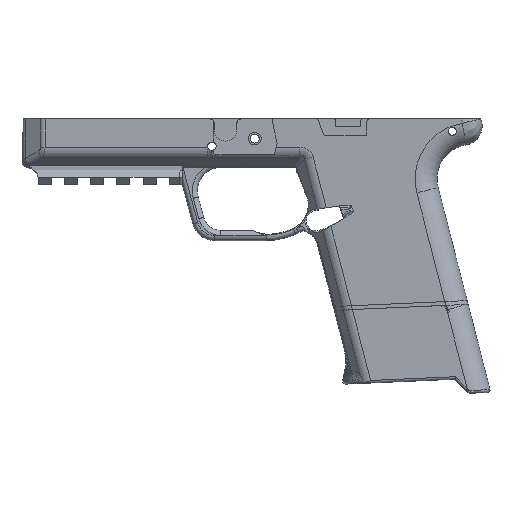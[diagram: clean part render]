
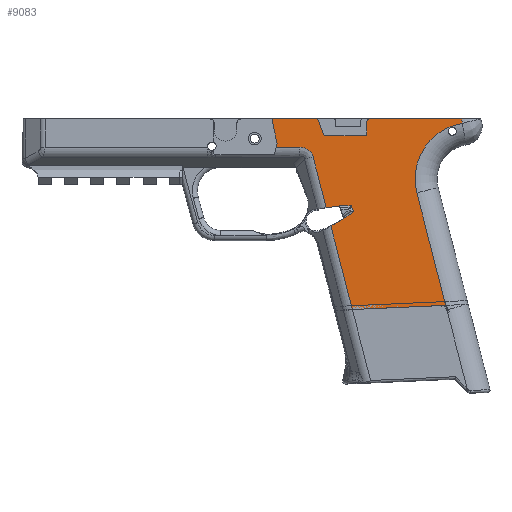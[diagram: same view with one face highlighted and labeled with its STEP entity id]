
A CAD part, left-side view. The second image highlights one B-rep face of the part: STEP entity #9083.
In plain terms, the highlighted face is planar.
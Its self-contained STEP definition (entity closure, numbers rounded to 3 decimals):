
#261=CIRCLE('',#9748,22.475);
#262=CIRCLE('',#9749,7.5);
#263=CIRCLE('',#9750,1.);
#264=CIRCLE('',#9751,1.);
#265=CIRCLE('',#9752,1.);
#266=CIRCLE('',#9753,1.);
#748=FACE_OUTER_BOUND('',#1268,.T.);
#1268=EDGE_LOOP('',(#6722,#6723,#6724,#6725,#6726,#6727,#6728,#6729,#6730,
#6731,#6732,#6733,#6734,#6735,#6736,#6737,#6738,#6739,#6740,#6741,#6742,
#6743,#6744,#6745,#6746,#6747));
#1880=LINE('',#14893,#2688);
#1882=LINE('',#14905,#2690);
#1884=LINE('',#14909,#2692);
#1895=LINE('',#14938,#2703);
#1896=LINE('',#14940,#2704);
#1897=LINE('',#14941,#2705);
#1898=LINE('',#14943,#2706);
#1899=LINE('',#14945,#2707);
#1900=LINE('',#14947,#2708);
#1901=LINE('',#14949,#2709);
#1902=LINE('',#14955,#2710);
#1903=LINE('',#14959,#2711);
#1904=LINE('',#14963,#2712);
#1905=LINE('',#14967,#2713);
#1906=LINE('',#14971,#2714);
#1907=LINE('',#14973,#2715);
#1908=LINE('',#14975,#2716);
#1909=LINE('',#14977,#2717);
#1910=LINE('',#14980,#2718);
#2688=VECTOR('',#11078,10.);
#2690=VECTOR('',#11088,10.);
#2692=VECTOR('',#11092,10.);
#2703=VECTOR('',#11113,10.);
#2704=VECTOR('',#11114,10.);
#2705=VECTOR('',#11115,10.);
#2706=VECTOR('',#11116,10.);
#2707=VECTOR('',#11117,10.);
#2708=VECTOR('',#11118,10.);
#2709=VECTOR('',#11119,10.);
#2710=VECTOR('',#11124,10.);
#2711=VECTOR('',#11127,10.);
#2712=VECTOR('',#11130,10.);
#2713=VECTOR('',#11133,10.);
#2714=VECTOR('',#11136,10.);
#2715=VECTOR('',#11137,10.);
#2716=VECTOR('',#11138,10.);
#2717=VECTOR('',#11139,10.);
#2718=VECTOR('',#11142,10.);
#3324=ELLIPSE('',#9754,10.693,7.);
#3900=VERTEX_POINT('',#14890);
#3901=VERTEX_POINT('',#14892);
#3906=VERTEX_POINT('',#14902);
#3907=VERTEX_POINT('',#14904);
#3908=VERTEX_POINT('',#14908);
#3921=VERTEX_POINT('',#14937);
#3922=VERTEX_POINT('',#14939);
#3923=VERTEX_POINT('',#14942);
#3924=VERTEX_POINT('',#14944);
#3925=VERTEX_POINT('',#14946);
#3926=VERTEX_POINT('',#14948);
#3927=VERTEX_POINT('',#14950);
#3928=VERTEX_POINT('',#14952);
#3929=VERTEX_POINT('',#14954);
#3930=VERTEX_POINT('',#14956);
#3931=VERTEX_POINT('',#14958);
#3932=VERTEX_POINT('',#14960);
#3933=VERTEX_POINT('',#14962);
#3934=VERTEX_POINT('',#14964);
#3935=VERTEX_POINT('',#14966);
#3936=VERTEX_POINT('',#14968);
#3937=VERTEX_POINT('',#14970);
#3938=VERTEX_POINT('',#14972);
#3939=VERTEX_POINT('',#14974);
#3940=VERTEX_POINT('',#14976);
#3941=VERTEX_POINT('',#14978);
#4934=EDGE_CURVE('',#3901,#3900,#1880,.T.);
#4940=EDGE_CURVE('',#3907,#3906,#1882,.T.);
#4942=EDGE_CURVE('',#3908,#3907,#1884,.T.);
#4957=EDGE_CURVE('',#3921,#3906,#1895,.T.);
#4958=EDGE_CURVE('',#3922,#3921,#1896,.T.);
#4959=EDGE_CURVE('',#3901,#3922,#1897,.T.);
#4960=EDGE_CURVE('',#3900,#3923,#1898,.T.);
#4961=EDGE_CURVE('',#3924,#3923,#1899,.T.);
#4962=EDGE_CURVE('',#3925,#3924,#1900,.T.);
#4963=EDGE_CURVE('',#3926,#3925,#1901,.T.);
#4964=EDGE_CURVE('',#3927,#3926,#261,.T.);
#4965=EDGE_CURVE('',#3928,#3927,#262,.T.);
#4966=EDGE_CURVE('',#3928,#3929,#1902,.T.);
#4967=EDGE_CURVE('',#3930,#3929,#263,.T.);
#4968=EDGE_CURVE('',#3930,#3931,#1903,.T.);
#4969=EDGE_CURVE('',#3932,#3931,#264,.T.);
#4970=EDGE_CURVE('',#3932,#3933,#1904,.T.);
#4971=EDGE_CURVE('',#3934,#3933,#265,.T.);
#4972=EDGE_CURVE('',#3935,#3934,#1905,.T.);
#4973=EDGE_CURVE('',#3936,#3935,#266,.T.);
#4974=EDGE_CURVE('',#3937,#3936,#1906,.T.);
#4975=EDGE_CURVE('',#3937,#3938,#1907,.T.);
#4976=EDGE_CURVE('',#3938,#3939,#1908,.T.);
#4977=EDGE_CURVE('',#3940,#3939,#1909,.T.);
#4978=EDGE_CURVE('',#3941,#3940,#3324,.T.);
#4979=EDGE_CURVE('',#3908,#3941,#1910,.T.);
#6722=ORIENTED_EDGE('',*,*,#4940,.T.);
#6723=ORIENTED_EDGE('',*,*,#4957,.F.);
#6724=ORIENTED_EDGE('',*,*,#4958,.F.);
#6725=ORIENTED_EDGE('',*,*,#4959,.F.);
#6726=ORIENTED_EDGE('',*,*,#4934,.T.);
#6727=ORIENTED_EDGE('',*,*,#4960,.T.);
#6728=ORIENTED_EDGE('',*,*,#4961,.F.);
#6729=ORIENTED_EDGE('',*,*,#4962,.F.);
#6730=ORIENTED_EDGE('',*,*,#4963,.F.);
#6731=ORIENTED_EDGE('',*,*,#4964,.F.);
#6732=ORIENTED_EDGE('',*,*,#4965,.F.);
#6733=ORIENTED_EDGE('',*,*,#4966,.T.);
#6734=ORIENTED_EDGE('',*,*,#4967,.F.);
#6735=ORIENTED_EDGE('',*,*,#4968,.T.);
#6736=ORIENTED_EDGE('',*,*,#4969,.F.);
#6737=ORIENTED_EDGE('',*,*,#4970,.T.);
#6738=ORIENTED_EDGE('',*,*,#4971,.F.);
#6739=ORIENTED_EDGE('',*,*,#4972,.F.);
#6740=ORIENTED_EDGE('',*,*,#4973,.F.);
#6741=ORIENTED_EDGE('',*,*,#4974,.F.);
#6742=ORIENTED_EDGE('',*,*,#4975,.T.);
#6743=ORIENTED_EDGE('',*,*,#4976,.T.);
#6744=ORIENTED_EDGE('',*,*,#4977,.F.);
#6745=ORIENTED_EDGE('',*,*,#4978,.F.);
#6746=ORIENTED_EDGE('',*,*,#4979,.F.);
#6747=ORIENTED_EDGE('',*,*,#4942,.T.);
#8756=PLANE('',#9747);
#9083=ADVANCED_FACE('',(#748),#8756,.F.);
#9747=AXIS2_PLACEMENT_3D('',#14936,#11111,#11112);
#9748=AXIS2_PLACEMENT_3D('',#14951,#11120,#11121);
#9749=AXIS2_PLACEMENT_3D('',#14953,#11122,#11123);
#9750=AXIS2_PLACEMENT_3D('',#14957,#11125,#11126);
#9751=AXIS2_PLACEMENT_3D('',#14961,#11128,#11129);
#9752=AXIS2_PLACEMENT_3D('',#14965,#11131,#11132);
#9753=AXIS2_PLACEMENT_3D('',#14969,#11134,#11135);
#9754=AXIS2_PLACEMENT_3D('',#14979,#11140,#11141);
#11078=DIRECTION('',(0.,-0.323,0.947));
#11088=DIRECTION('',(0.,-0.323,0.947));
#11092=DIRECTION('',(0.,-0.991,-0.136));
#11111=DIRECTION('center_axis',(-1.,0.,0.));
#11112=DIRECTION('ref_axis',(0.,1.,0.));
#11113=DIRECTION('',(0.,0.998,0.056));
#11114=DIRECTION('',(0.,0.323,-0.947));
#11115=DIRECTION('',(0.,-0.828,-0.56));
#11116=DIRECTION('',(0.,0.87,0.492));
#11117=DIRECTION('',(0.,0.249,-0.969));
#11118=DIRECTION('',(0.,0.999,0.044));
#11119=DIRECTION('',(0.,-0.249,0.969));
#11120=DIRECTION('center_axis',(1.,0.,0.));
#11121=DIRECTION('ref_axis',(0.,0.,1.));
#11122=DIRECTION('center_axis',(1.,0.,0.));
#11123=DIRECTION('ref_axis',(0.,-0.97,-0.244));
#11124=DIRECTION('',(0.,1.,0.));
#11125=DIRECTION('center_axis',(-1.,0.,0.));
#11126=DIRECTION('ref_axis',(0.,0.707,-0.707));
#11127=DIRECTION('',(0.,0.,1.));
#11128=DIRECTION('center_axis',(1.,0.,0.));
#11129=DIRECTION('ref_axis',(0.,-0.707,0.707));
#11130=DIRECTION('',(0.,1.,0.));
#11131=DIRECTION('center_axis',(1.,0.,0.));
#11132=DIRECTION('ref_axis',(0.,0.576,0.817));
#11133=DIRECTION('',(0.,-0.336,0.942));
#11134=DIRECTION('center_axis',(-1.,0.,0.));
#11135=DIRECTION('ref_axis',(0.,-0.576,-0.817));
#11136=DIRECTION('',(0.,-1.,0.));
#11137=DIRECTION('',(0.,-0.21,0.978));
#11138=DIRECTION('',(0.,0.21,0.978));
#11139=DIRECTION('',(0.,1.,0.));
#11140=DIRECTION('center_axis',(1.,0.,0.));
#11141=DIRECTION('ref_axis',(0.,-0.714,-0.7));
#11142=DIRECTION('',(0.,0.249,-0.969));
#14890=CARTESIAN_POINT('',(22.175,-34.01,32.318));
#14892=CARTESIAN_POINT('',(22.175,-33.995,32.275));
#14893=CARTESIAN_POINT('',(22.175,-27.197,12.322));
#14902=CARTESIAN_POINT('',(22.175,-32.296,27.288));
#14904=CARTESIAN_POINT('',(22.175,-32.284,27.253));
#14905=CARTESIAN_POINT('',(22.175,-27.197,12.322));
#14908=CARTESIAN_POINT('',(22.175,-27.009,27.98));
#14909=CARTESIAN_POINT('',(22.175,-17.622,29.272));
#14936=CARTESIAN_POINT('Origin',(22.175,-7.921,2.186));
#14937=CARTESIAN_POINT('',(22.175,-36.962,27.028));
#14938=CARTESIAN_POINT('',(22.175,-22.893,27.813));
#14939=CARTESIAN_POINT('',(22.175,-37.859,29.661));
#14940=CARTESIAN_POINT('',(22.175,-32.016,12.512));
#14941=CARTESIAN_POINT('',(22.175,-30.049,34.945));
#14942=CARTESIAN_POINT('',(22.175,-28.871,35.225));
#14943=CARTESIAN_POINT('',(22.175,-30.348,34.389));
#14944=CARTESIAN_POINT('',(22.175,-37.447,68.587));
#14945=CARTESIAN_POINT('',(22.175,-26.659,26.619));
#14946=CARTESIAN_POINT('',(22.175,-74.722,66.935));
#14947=CARTESIAN_POINT('',(22.175,-40.785,68.439));
#14948=CARTESIAN_POINT('',(22.175,-63.184,22.049));
#14949=CARTESIAN_POINT('',(22.175,-75.103,68.418));
#14950=CARTESIAN_POINT('',(22.175,-81.332,-5.728));
#14951=CARTESIAN_POINT('Origin',(22.175,-84.951,16.453));
#14952=CARTESIAN_POINT('',(22.175,-81.106,-7.556));
#14953=CARTESIAN_POINT('Origin',(22.175,-88.606,-7.556));
#14954=CARTESIAN_POINT('',(22.175,-44.284,-7.556));
#14955=CARTESIAN_POINT('',(22.175,-84.951,-7.556));
#14956=CARTESIAN_POINT('',(22.175,-43.284,-6.556));
#14957=CARTESIAN_POINT('Origin',(22.175,-44.284,-6.556));
#14958=CARTESIAN_POINT('',(22.175,-43.284,-1.806));
#14959=CARTESIAN_POINT('',(22.175,-43.284,-2.685));
#14960=CARTESIAN_POINT('',(22.175,-42.284,-0.806));
#14961=CARTESIAN_POINT('Origin',(22.175,-42.284,-1.806));
#14962=CARTESIAN_POINT('',(22.175,-26.754,-0.806));
#14963=CARTESIAN_POINT('',(22.175,-30.774,-0.806));
#14964=CARTESIAN_POINT('',(22.175,-25.812,-1.47));
#14965=CARTESIAN_POINT('Origin',(22.175,-26.754,-1.806));
#14966=CARTESIAN_POINT('',(22.175,-23.877,-6.892));
#14967=CARTESIAN_POINT('',(22.175,-23.64,-7.556));
#14968=CARTESIAN_POINT('',(22.175,-22.935,-7.556));
#14969=CARTESIAN_POINT('Origin',(22.175,-22.935,-6.556));
#14970=CARTESIAN_POINT('',(22.175,-5.3,-7.556));
#14971=CARTESIAN_POINT('',(22.175,-8.213,-7.556));
#14972=CARTESIAN_POINT('',(22.175,-7.389,2.186));
#14973=CARTESIAN_POINT('',(22.175,-6.356,-2.63));
#14974=CARTESIAN_POINT('',(22.175,-7.025,3.884));
#14975=CARTESIAN_POINT('',(22.175,-7.4,2.132));
#14976=CARTESIAN_POINT('',(22.175,-16.536,3.884));
#14977=CARTESIAN_POINT('',(22.175,33.814,3.884));
#14978=CARTESIAN_POINT('',(22.175,-21.783,7.651));
#14979=CARTESIAN_POINT('Origin',(22.175,-12.907,12.884));
#14980=CARTESIAN_POINT('',(22.175,-26.659,26.619));
